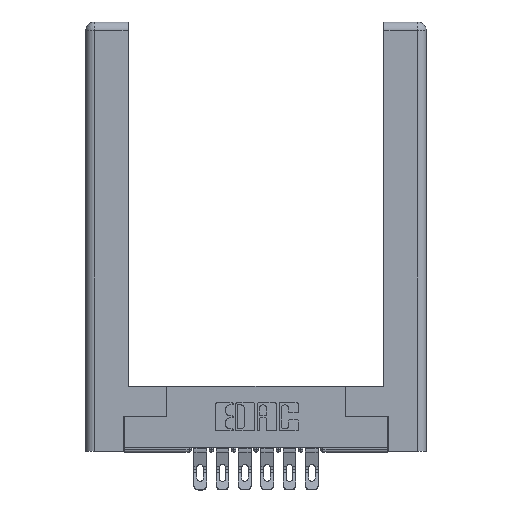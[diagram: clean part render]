
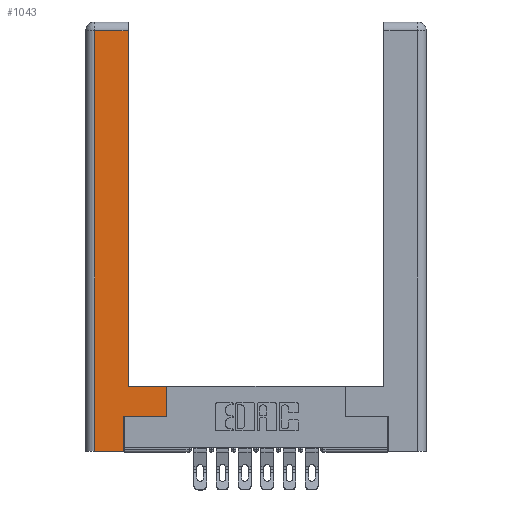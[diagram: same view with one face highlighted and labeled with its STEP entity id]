
A CAD part, top view. The second image highlights one B-rep face of the part: STEP entity #1043.
In plain terms, the highlighted planar face has unit normal (0, 0, 1).
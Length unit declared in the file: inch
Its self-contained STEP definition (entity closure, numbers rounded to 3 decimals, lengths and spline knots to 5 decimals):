
#327 = VERTEX_POINT ( 'NONE', #1834 ) ;
#971 = DIRECTION ( 'NONE',  ( 1., 0., 0. ) ) ;
#1043 = ADVANCED_FACE ( 'NONE', ( #7510 ), #10795, .F. ) ;
#1086 = VECTOR ( 'NONE', #13964, 39.37008 ) ;
#1106 = VERTEX_POINT ( 'NONE', #12012 ) ;
#1173 = CARTESIAN_POINT ( 'NONE',  ( 0.265, 0., 0. ) ) ;
#1661 = EDGE_CURVE ( 'NONE', #2998, #13815, #6292, .T. ) ;
#1834 = CARTESIAN_POINT ( 'NONE',  ( 0.295, 2.94, 0. ) ) ;
#1875 = CARTESIAN_POINT ( 'NONE',  ( 0.565, 0.245, 0. ) ) ;
#2122 = EDGE_LOOP ( 'NONE', ( #7000, #3557, #11082, #9778, #5317, #4359, #5462, #5634 ) ) ;
#2777 = VECTOR ( 'NONE', #5145, 39.37008 ) ;
#2831 = EDGE_CURVE ( 'NONE', #12924, #6673, #13290, .T. ) ;
#2998 = VERTEX_POINT ( 'NONE', #8100 ) ;
#3259 = LINE ( 'NONE', #3610, #10811 ) ;
#3404 = VECTOR ( 'NONE', #10776, 39.37008 ) ;
#3557 = ORIENTED_EDGE ( 'NONE', *, *, #4461, .T. ) ;
#3610 = CARTESIAN_POINT ( 'NONE',  ( 0.265, 0.245, 0. ) ) ;
#4121 = DIRECTION ( 'NONE',  ( -1., 0., 0. ) ) ;
#4356 = DIRECTION ( 'NONE',  ( 0., 1., 0. ) ) ;
#4359 = ORIENTED_EDGE ( 'NONE', *, *, #12033, .T. ) ;
#4384 = CARTESIAN_POINT ( 'NONE',  ( 0.0615, 2.94, 0. ) ) ;
#4456 = CARTESIAN_POINT ( 'NONE',  ( 0.0615, 0., 0. ) ) ;
#4461 = EDGE_CURVE ( 'NONE', #327, #12924, #5536, .T. ) ;
#5098 = CARTESIAN_POINT ( 'NONE',  ( 0., 0., 0. ) ) ;
#5145 = DIRECTION ( 'NONE',  ( 0., 1., 0. ) ) ;
#5317 = ORIENTED_EDGE ( 'NONE', *, *, #6326, .T. ) ;
#5359 = CARTESIAN_POINT ( 'NONE',  ( 0.265, 0., 0. ) ) ;
#5462 = ORIENTED_EDGE ( 'NONE', *, *, #8338, .T. ) ;
#5536 = LINE ( 'NONE', #9515, #6217 ) ;
#5634 = ORIENTED_EDGE ( 'NONE', *, *, #1661, .T. ) ;
#5758 = VECTOR ( 'NONE', #7750, 39.37008 ) ;
#5968 = VERTEX_POINT ( 'NONE', #1173 ) ;
#6217 = VECTOR ( 'NONE', #12797, 39.37008 ) ;
#6292 = LINE ( 'NONE', #6349, #3404 ) ;
#6326 = EDGE_CURVE ( 'NONE', #5968, #1106, #3259, .T. ) ;
#6349 = CARTESIAN_POINT ( 'NONE',  ( 0.295, 0.45, 0. ) ) ;
#6471 = CARTESIAN_POINT ( 'NONE',  ( 0.295, 0.45, 0. ) ) ;
#6673 = VERTEX_POINT ( 'NONE', #11035 ) ;
#7000 = ORIENTED_EDGE ( 'NONE', *, *, #12250, .T. ) ;
#7494 = VERTEX_POINT ( 'NONE', #1875 ) ;
#7510 = FACE_OUTER_BOUND ( 'NONE', #2122, .T. ) ;
#7692 = CARTESIAN_POINT ( 'NONE',  ( 0.565, 0.245, 0. ) ) ;
#7750 = DIRECTION ( 'NONE',  ( 0., -1., 0. ) ) ;
#8100 = CARTESIAN_POINT ( 'NONE',  ( 0.565, 0.45, 0. ) ) ;
#8331 = EDGE_CURVE ( 'NONE', #6673, #5968, #10145, .T. ) ;
#8338 = EDGE_CURVE ( 'NONE', #7494, #2998, #12016, .T. ) ;
#8661 = VECTOR ( 'NONE', #971, 39.37008 ) ;
#9184 = LINE ( 'NONE', #9731, #10722 ) ;
#9515 = CARTESIAN_POINT ( 'NONE',  ( 0.0615, 2.94, 0. ) ) ;
#9731 = CARTESIAN_POINT ( 'NONE',  ( 0.295, 3., 0. ) ) ;
#9778 = ORIENTED_EDGE ( 'NONE', *, *, #8331, .T. ) ;
#10145 = LINE ( 'NONE', #5359, #1086 ) ;
#10722 = VECTOR ( 'NONE', #12087, 39.37008 ) ;
#10776 = DIRECTION ( 'NONE',  ( -1., 0., 0. ) ) ;
#10795 = PLANE ( 'NONE',  #12785 ) ;
#10811 = VECTOR ( 'NONE', #4356, 39.37008 ) ;
#11035 = CARTESIAN_POINT ( 'NONE',  ( 0.0615, 0., 0. ) ) ;
#11082 = ORIENTED_EDGE ( 'NONE', *, *, #2831, .T. ) ;
#11725 = CARTESIAN_POINT ( 'NONE',  ( 0.565, 0.45, 0. ) ) ;
#12012 = CARTESIAN_POINT ( 'NONE',  ( 0.265, 0.245, 0. ) ) ;
#12016 = LINE ( 'NONE', #11725, #2777 ) ;
#12033 = EDGE_CURVE ( 'NONE', #1106, #7494, #12941, .T. ) ;
#12087 = DIRECTION ( 'NONE',  ( 0., 1., 0. ) ) ;
#12250 = EDGE_CURVE ( 'NONE', #13815, #327, #9184, .T. ) ;
#12718 = DIRECTION ( 'NONE',  ( 0., 0., -1. ) ) ;
#12785 = AXIS2_PLACEMENT_3D ( 'NONE', #5098, #12718, #4121 ) ;
#12797 = DIRECTION ( 'NONE',  ( -1., 0., 0. ) ) ;
#12924 = VERTEX_POINT ( 'NONE', #4384 ) ;
#12941 = LINE ( 'NONE', #7692, #8661 ) ;
#13290 = LINE ( 'NONE', #4456, #5758 ) ;
#13815 = VERTEX_POINT ( 'NONE', #6471 ) ;
#13964 = DIRECTION ( 'NONE',  ( 1., 0., 0. ) ) ;
